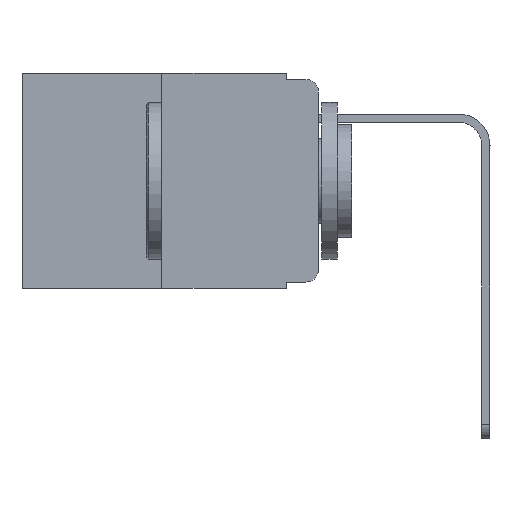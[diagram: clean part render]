
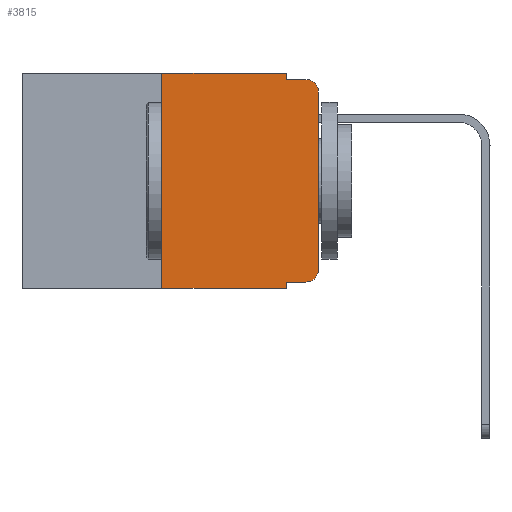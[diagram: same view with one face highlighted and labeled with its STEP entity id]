
A CAD part, left-side view. The second image highlights one B-rep face of the part: STEP entity #3815.
In plain terms, the highlighted planar face has unit normal (-1, 0, 0).
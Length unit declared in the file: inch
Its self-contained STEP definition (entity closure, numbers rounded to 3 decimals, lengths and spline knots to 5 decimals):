
#62 = CIRCLE ( 'NONE', #2539, 0.02 ) ;
#127 = EDGE_CURVE ( 'NONE', #11144, #7564, #163, .T. ) ;
#163 = CIRCLE ( 'NONE', #9756, 0.02 ) ;
#188 = EDGE_CURVE ( 'NONE', #871, #2839, #10996, .T. ) ;
#204 = DIRECTION ( 'NONE',  ( -1., 0., 0. ) ) ;
#404 = ORIENTED_EDGE ( 'NONE', *, *, #2874, .F. ) ;
#643 = AXIS2_PLACEMENT_3D ( 'NONE', #6036, #8721, #1614 ) ;
#871 = VERTEX_POINT ( 'NONE', #5979 ) ;
#939 = CARTESIAN_POINT ( 'NONE',  ( 0., 0., -0.313 ) ) ;
#1252 = CARTESIAN_POINT ( 'NONE',  ( 0., 0.051, -0.343 ) ) ;
#1526 = FACE_OUTER_BOUND ( 'NONE', #7779, .T. ) ;
#1560 = VECTOR ( 'NONE', #5689, 39.37008 ) ;
#1614 = DIRECTION ( 'NONE',  ( 0., 0., -1. ) ) ;
#1960 = VECTOR ( 'NONE', #3496, 39.37008 ) ;
#2102 = LINE ( 'NONE', #4301, #5602 ) ;
#2368 = LINE ( 'NONE', #6373, #8747 ) ;
#2539 = AXIS2_PLACEMENT_3D ( 'NONE', #4084, #11161, #5830 ) ;
#2557 = DIRECTION ( 'NONE',  ( 0., -1., 0. ) ) ;
#2614 = EDGE_CURVE ( 'NONE', #7143, #11144, #2102, .T. ) ;
#2641 = VERTEX_POINT ( 'NONE', #3296 ) ;
#2839 = VERTEX_POINT ( 'NONE', #4682 ) ;
#2874 = EDGE_CURVE ( 'NONE', #2641, #6081, #4227, .T. ) ;
#2949 = ORIENTED_EDGE ( 'NONE', *, *, #7808, .T. ) ;
#2978 = VERTEX_POINT ( 'NONE', #9266 ) ;
#3296 = CARTESIAN_POINT ( 'NONE',  ( 0., 0.051, 0. ) ) ;
#3496 = DIRECTION ( 'NONE',  ( 0., 0., 1. ) ) ;
#3815 = ADVANCED_FACE ( 'NONE', ( #1526 ), #11328, .F. ) ;
#4084 = CARTESIAN_POINT ( 'NONE',  ( 0., 0.02, -0.03 ) ) ;
#4223 = ORIENTED_EDGE ( 'NONE', *, *, #5723, .F. ) ;
#4227 = LINE ( 'NONE', #8273, #10311 ) ;
#4259 = VERTEX_POINT ( 'NONE', #1252 ) ;
#4301 = CARTESIAN_POINT ( 'NONE',  ( 0., 0.051, -0.333 ) ) ;
#4682 = CARTESIAN_POINT ( 'NONE',  ( 0., 0.25, 0. ) ) ;
#4985 = CARTESIAN_POINT ( 'NONE',  ( 0., 0.051, -0.333 ) ) ;
#5483 = DIRECTION ( 'NONE',  ( 0., 0., -1. ) ) ;
#5522 = CARTESIAN_POINT ( 'NONE',  ( 0., 0.051, -0.01 ) ) ;
#5602 = VECTOR ( 'NONE', #2557, 39.37008 ) ;
#5608 = DIRECTION ( 'NONE',  ( 0., -1., 0. ) ) ;
#5632 = ORIENTED_EDGE ( 'NONE', *, *, #2614, .T. ) ;
#5689 = DIRECTION ( 'NONE',  ( 0., 0., -1. ) ) ;
#5723 = EDGE_CURVE ( 'NONE', #2839, #2641, #2368, .T. ) ;
#5830 = DIRECTION ( 'NONE',  ( 0., 0., -1. ) ) ;
#5929 = CARTESIAN_POINT ( 'NONE',  ( 0., 0.051, -0.01 ) ) ;
#5979 = CARTESIAN_POINT ( 'NONE',  ( 0., 0.25, -0.343 ) ) ;
#5991 = DIRECTION ( 'NONE',  ( 0., -1., 0. ) ) ;
#6031 = CARTESIAN_POINT ( 'NONE',  ( 0., 0.473, -0.343 ) ) ;
#6036 = CARTESIAN_POINT ( 'NONE',  ( 0., 0.473, 0. ) ) ;
#6081 = VERTEX_POINT ( 'NONE', #5929 ) ;
#6286 = ORIENTED_EDGE ( 'NONE', *, *, #10878, .T. ) ;
#6327 = LINE ( 'NONE', #10989, #1560 ) ;
#6373 = CARTESIAN_POINT ( 'NONE',  ( 0., 0.473, 0. ) ) ;
#6447 = ORIENTED_EDGE ( 'NONE', *, *, #10567, .F. ) ;
#6509 = DIRECTION ( 'NONE',  ( 0., -1., 0. ) ) ;
#6630 = VERTEX_POINT ( 'NONE', #10401 ) ;
#6733 = ORIENTED_EDGE ( 'NONE', *, *, #8425, .F. ) ;
#6983 = ORIENTED_EDGE ( 'NONE', *, *, #188, .F. ) ;
#6985 = VECTOR ( 'NONE', #10486, 39.37008 ) ;
#7143 = VERTEX_POINT ( 'NONE', #4985 ) ;
#7349 = CARTESIAN_POINT ( 'NONE',  ( 0., 0.02, -0.333 ) ) ;
#7564 = VERTEX_POINT ( 'NONE', #939 ) ;
#7594 = ORIENTED_EDGE ( 'NONE', *, *, #10342, .T. ) ;
#7779 = EDGE_LOOP ( 'NONE', ( #7594, #2949, #6447, #404, #4223, #6983, #6286, #6733, #5632, #8957 ) ) ;
#7808 = EDGE_CURVE ( 'NONE', #2978, #6630, #62, .T. ) ;
#7813 = CARTESIAN_POINT ( 'NONE',  ( 0., 0.25, 0. ) ) ;
#8273 = CARTESIAN_POINT ( 'NONE',  ( 0., 0.051, 0. ) ) ;
#8425 = EDGE_CURVE ( 'NONE', #7143, #4259, #6327, .T. ) ;
#8481 = LINE ( 'NONE', #6031, #9020 ) ;
#8721 = DIRECTION ( 'NONE',  ( 1., 0., 0. ) ) ;
#8747 = VECTOR ( 'NONE', #5608, 39.37008 ) ;
#8904 = LINE ( 'NONE', #11476, #6985 ) ;
#8957 = ORIENTED_EDGE ( 'NONE', *, *, #127, .T. ) ;
#9020 = VECTOR ( 'NONE', #5991, 39.37008 ) ;
#9266 = CARTESIAN_POINT ( 'NONE',  ( 0., 0., -0.03 ) ) ;
#9723 = LINE ( 'NONE', #5522, #10282 ) ;
#9756 = AXIS2_PLACEMENT_3D ( 'NONE', #9912, #204, #9868 ) ;
#9868 = DIRECTION ( 'NONE',  ( 0., 0., -1. ) ) ;
#9912 = CARTESIAN_POINT ( 'NONE',  ( 0., 0.02, -0.313 ) ) ;
#10282 = VECTOR ( 'NONE', #6509, 39.37008 ) ;
#10311 = VECTOR ( 'NONE', #5483, 39.37008 ) ;
#10342 = EDGE_CURVE ( 'NONE', #7564, #2978, #8904, .T. ) ;
#10401 = CARTESIAN_POINT ( 'NONE',  ( 0., 0.02, -0.01 ) ) ;
#10486 = DIRECTION ( 'NONE',  ( 0., 0., 1. ) ) ;
#10567 = EDGE_CURVE ( 'NONE', #6081, #6630, #9723, .T. ) ;
#10878 = EDGE_CURVE ( 'NONE', #871, #4259, #8481, .T. ) ;
#10989 = CARTESIAN_POINT ( 'NONE',  ( 0., 0.051, 0. ) ) ;
#10996 = LINE ( 'NONE', #7813, #1960 ) ;
#11144 = VERTEX_POINT ( 'NONE', #7349 ) ;
#11161 = DIRECTION ( 'NONE',  ( -1., 0., 0. ) ) ;
#11328 = PLANE ( 'NONE',  #643 ) ;
#11476 = CARTESIAN_POINT ( 'NONE',  ( 0., 0., 0. ) ) ;
